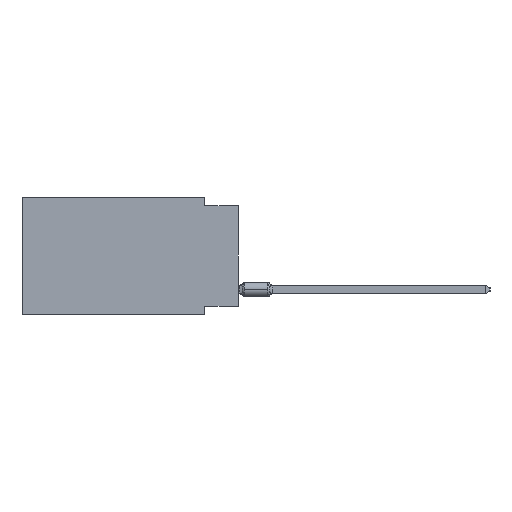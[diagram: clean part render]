
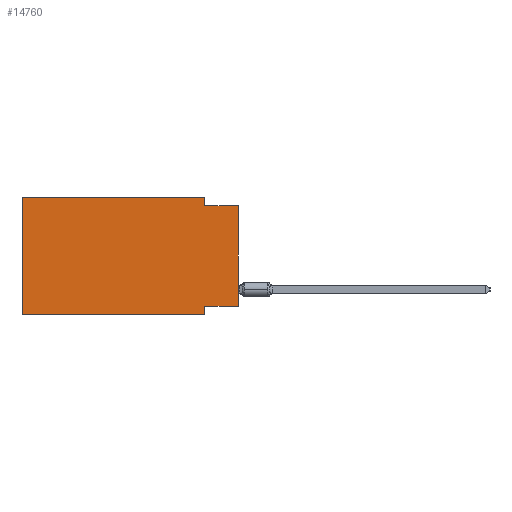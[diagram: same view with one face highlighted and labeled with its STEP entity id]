
A CAD part, left-side view. The second image highlights one B-rep face of the part: STEP entity #14760.
In plain terms, the highlighted planar face has unit normal (-1, 0, 0).
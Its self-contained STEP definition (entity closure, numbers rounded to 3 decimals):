
#108 = LINE ( 'NONE', #60564, #54751 ) ;
#1614 = CARTESIAN_POINT ( 'NONE',  ( 0., 16.383, -8.89 ) ) ;
#3369 = VERTEX_POINT ( 'NONE', #33942 ) ;
#3909 = VERTEX_POINT ( 'NONE', #69802 ) ;
#5173 = EDGE_CURVE ( 'NONE', #16972, #12144, #81233, .T. ) ;
#6493 = VERTEX_POINT ( 'NONE', #64721 ) ;
#7268 = CARTESIAN_POINT ( 'NONE',  ( 0., 2.54, -8.255 ) ) ;
#8603 = DIRECTION ( 'NONE',  ( 0., -1., 0. ) ) ;
#11862 = VERTEX_POINT ( 'NONE', #66474 ) ;
#12144 = VERTEX_POINT ( 'NONE', #65098 ) ;
#13145 = DIRECTION ( 'NONE',  ( 0., 0., 1. ) ) ;
#14248 = PLANE ( 'NONE',  #23786 ) ;
#14760 = ADVANCED_FACE ( 'NONE', ( #47326 ), #14248, .F. ) ;
#15198 = DIRECTION ( 'NONE',  ( 0., -1., 0. ) ) ;
#16357 = EDGE_CURVE ( 'NONE', #11862, #3369, #25264, .T. ) ;
#16966 = VECTOR ( 'NONE', #52230, 1000. ) ;
#16972 = VERTEX_POINT ( 'NONE', #1614 ) ;
#19713 = LINE ( 'NONE', #67552, #75814 ) ;
#19991 = EDGE_CURVE ( 'NONE', #3909, #67336, #33871, .T. ) ;
#23786 = AXIS2_PLACEMENT_3D ( 'NONE', #34272, #70543, #77918 ) ;
#25264 = LINE ( 'NONE', #45707, #16966 ) ;
#28350 = DIRECTION ( 'NONE',  ( 0., 0., -1. ) ) ;
#29285 = EDGE_CURVE ( 'NONE', #6493, #3909, #34363, .T. ) ;
#30006 = VECTOR ( 'NONE', #46930, 1000. ) ;
#32239 = VECTOR ( 'NONE', #8603, 1000. ) ;
#33871 = LINE ( 'NONE', #40830, #30006 ) ;
#33942 = CARTESIAN_POINT ( 'NONE',  ( 0., 0., -0.635 ) ) ;
#34272 = CARTESIAN_POINT ( 'NONE',  ( 0., 16.383, 0. ) ) ;
#34363 = LINE ( 'NONE', #80891, #69819 ) ;
#37112 = ORIENTED_EDGE ( 'NONE', *, *, #76721, .F. ) ;
#38610 = ORIENTED_EDGE ( 'NONE', *, *, #16357, .T. ) ;
#39294 = DIRECTION ( 'NONE',  ( 0., 1., 0. ) ) ;
#40183 = EDGE_LOOP ( 'NONE', ( #38610, #76744, #58252, #82656, #40262, #58688, #44221, #37112 ) ) ;
#40262 = ORIENTED_EDGE ( 'NONE', *, *, #75583, .F. ) ;
#40830 = CARTESIAN_POINT ( 'NONE',  ( 0., 2.54, 0. ) ) ;
#41669 = CARTESIAN_POINT ( 'NONE',  ( 0., 16.383, -8.89 ) ) ;
#41832 = LINE ( 'NONE', #54450, #45445 ) ;
#43872 = EDGE_CURVE ( 'NONE', #67336, #3369, #19713, .T. ) ;
#44221 = ORIENTED_EDGE ( 'NONE', *, *, #55036, .F. ) ;
#45445 = VECTOR ( 'NONE', #28350, 1000. ) ;
#45707 = CARTESIAN_POINT ( 'NONE',  ( 0., 0., 0. ) ) ;
#46930 = DIRECTION ( 'NONE',  ( 0., 0., -1. ) ) ;
#47326 = FACE_OUTER_BOUND ( 'NONE', #40183, .T. ) ;
#52230 = DIRECTION ( 'NONE',  ( 0., 0., 1. ) ) ;
#54450 = CARTESIAN_POINT ( 'NONE',  ( 0., 2.54, -8.89 ) ) ;
#54751 = VECTOR ( 'NONE', #13145, 1000. ) ;
#55036 = EDGE_CURVE ( 'NONE', #55674, #12144, #41832, .T. ) ;
#55674 = VERTEX_POINT ( 'NONE', #7268 ) ;
#58252 = ORIENTED_EDGE ( 'NONE', *, *, #19991, .F. ) ;
#58434 = LINE ( 'NONE', #71920, #73743 ) ;
#58688 = ORIENTED_EDGE ( 'NONE', *, *, #5173, .T. ) ;
#60564 = CARTESIAN_POINT ( 'NONE',  ( 0., 16.383, 0. ) ) ;
#64721 = CARTESIAN_POINT ( 'NONE',  ( 0., 16.383, 0. ) ) ;
#65098 = CARTESIAN_POINT ( 'NONE',  ( 0., 2.54, -8.89 ) ) ;
#66474 = CARTESIAN_POINT ( 'NONE',  ( 0., 0., -8.255 ) ) ;
#67135 = DIRECTION ( 'NONE',  ( 0., -1., 0. ) ) ;
#67336 = VERTEX_POINT ( 'NONE', #70156 ) ;
#67552 = CARTESIAN_POINT ( 'NONE',  ( 0., 0., -0.635 ) ) ;
#69802 = CARTESIAN_POINT ( 'NONE',  ( 0., 2.54, 0. ) ) ;
#69819 = VECTOR ( 'NONE', #15198, 1000. ) ;
#70156 = CARTESIAN_POINT ( 'NONE',  ( 0., 2.54, -0.635 ) ) ;
#70543 = DIRECTION ( 'NONE',  ( 1., 0., 0. ) ) ;
#71920 = CARTESIAN_POINT ( 'NONE',  ( 0., 0., -8.255 ) ) ;
#73743 = VECTOR ( 'NONE', #39294, 1000. ) ;
#75583 = EDGE_CURVE ( 'NONE', #16972, #6493, #108, .T. ) ;
#75814 = VECTOR ( 'NONE', #67135, 1000. ) ;
#76721 = EDGE_CURVE ( 'NONE', #11862, #55674, #58434, .T. ) ;
#76744 = ORIENTED_EDGE ( 'NONE', *, *, #43872, .F. ) ;
#77918 = DIRECTION ( 'NONE',  ( 0., 0., -1. ) ) ;
#80891 = CARTESIAN_POINT ( 'NONE',  ( 0., 16.383, 0. ) ) ;
#81233 = LINE ( 'NONE', #41669, #32239 ) ;
#82656 = ORIENTED_EDGE ( 'NONE', *, *, #29285, .F. ) ;
